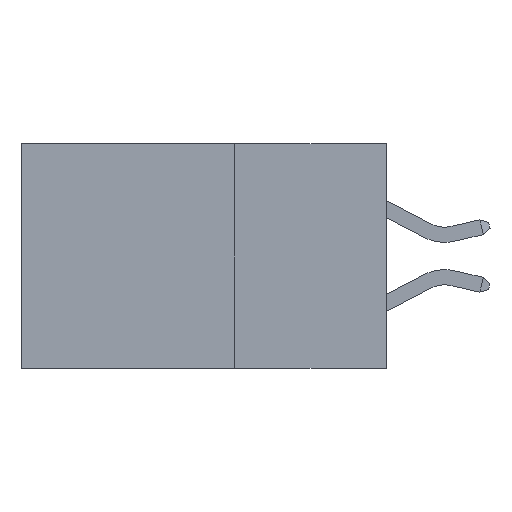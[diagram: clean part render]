
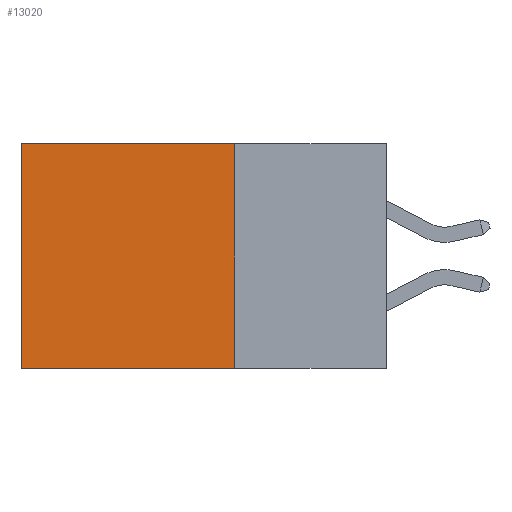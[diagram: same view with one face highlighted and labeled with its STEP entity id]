
A CAD part, left-side view. The second image highlights one B-rep face of the part: STEP entity #13020.
In plain terms, the highlighted planar face has unit normal (-1, 0, 0).
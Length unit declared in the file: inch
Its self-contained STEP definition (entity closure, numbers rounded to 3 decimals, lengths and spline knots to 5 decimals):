
#283 = VERTEX_POINT ( 'NONE', #4337 ) ;
#643 = CARTESIAN_POINT ( 'NONE',  ( 0.2615, 0.25, 0. ) ) ;
#716 = VERTEX_POINT ( 'NONE', #13739 ) ;
#719 = VECTOR ( 'NONE', #12884, 39.37008 ) ;
#821 = ORIENTED_EDGE ( 'NONE', *, *, #12348, .T. ) ;
#889 = LINE ( 'NONE', #5722, #5248 ) ;
#1500 = LINE ( 'NONE', #643, #11586 ) ;
#2637 = EDGE_CURVE ( 'NONE', #283, #716, #889, .T. ) ;
#3311 = CARTESIAN_POINT ( 'NONE',  ( 0.2615, 0.25, -0.37 ) ) ;
#3648 = VECTOR ( 'NONE', #10119, 39.37008 ) ;
#4337 = CARTESIAN_POINT ( 'NONE',  ( 0.2615, 0.6, 0. ) ) ;
#4364 = EDGE_LOOP ( 'NONE', ( #12932, #11219, #12339, #821 ) ) ;
#5248 = VECTOR ( 'NONE', #13012, 39.37008 ) ;
#5722 = CARTESIAN_POINT ( 'NONE',  ( 0.2615, 0.6, -0.37 ) ) ;
#6426 = LINE ( 'NONE', #10192, #3648 ) ;
#6502 = CARTESIAN_POINT ( 'NONE',  ( 0.2615, 0.25, -0.37 ) ) ;
#6748 = FACE_OUTER_BOUND ( 'NONE', #4364, .T. ) ;
#7417 = VERTEX_POINT ( 'NONE', #6502 ) ;
#8007 = DIRECTION ( 'NONE',  ( 1., 0., 0. ) ) ;
#8181 = CARTESIAN_POINT ( 'NONE',  ( 0.2615, 0.25, 0. ) ) ;
#9184 = CARTESIAN_POINT ( 'NONE',  ( 0.2615, 0.25, -0.37 ) ) ;
#9334 = LINE ( 'NONE', #3311, #719 ) ;
#9636 = EDGE_CURVE ( 'NONE', #7417, #716, #6426, .T. ) ;
#9696 = AXIS2_PLACEMENT_3D ( 'NONE', #9184, #8007, #10588 ) ;
#10119 = DIRECTION ( 'NONE',  ( 0., 1., 0. ) ) ;
#10192 = CARTESIAN_POINT ( 'NONE',  ( 0.2615, 0.25, -0.37 ) ) ;
#10588 = DIRECTION ( 'NONE',  ( 0., 0., -1. ) ) ;
#11219 = ORIENTED_EDGE ( 'NONE', *, *, #9636, .F. ) ;
#11586 = VECTOR ( 'NONE', #13477, 39.37008 ) ;
#11842 = VERTEX_POINT ( 'NONE', #8181 ) ;
#12339 = ORIENTED_EDGE ( 'NONE', *, *, #13041, .F. ) ;
#12348 = EDGE_CURVE ( 'NONE', #11842, #283, #1500, .T. ) ;
#12884 = DIRECTION ( 'NONE',  ( 0., 0., -1. ) ) ;
#12932 = ORIENTED_EDGE ( 'NONE', *, *, #2637, .T. ) ;
#13012 = DIRECTION ( 'NONE',  ( 0., 0., -1. ) ) ;
#13020 = ADVANCED_FACE ( 'NONE', ( #6748 ), #15303, .F. ) ;
#13041 = EDGE_CURVE ( 'NONE', #11842, #7417, #9334, .T. ) ;
#13477 = DIRECTION ( 'NONE',  ( 0., 1., 0. ) ) ;
#13739 = CARTESIAN_POINT ( 'NONE',  ( 0.2615, 0.6, -0.37 ) ) ;
#15303 = PLANE ( 'NONE',  #9696 ) ;
